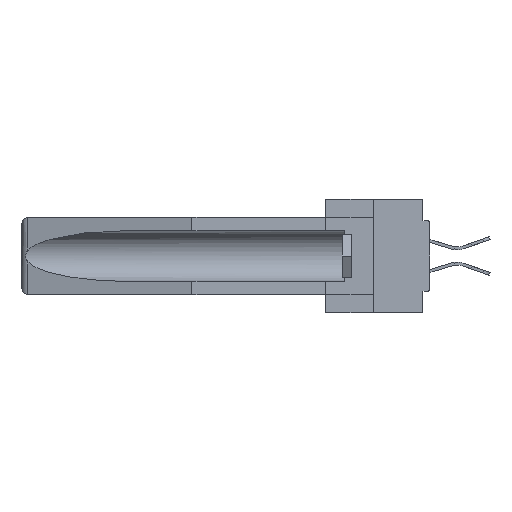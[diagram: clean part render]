
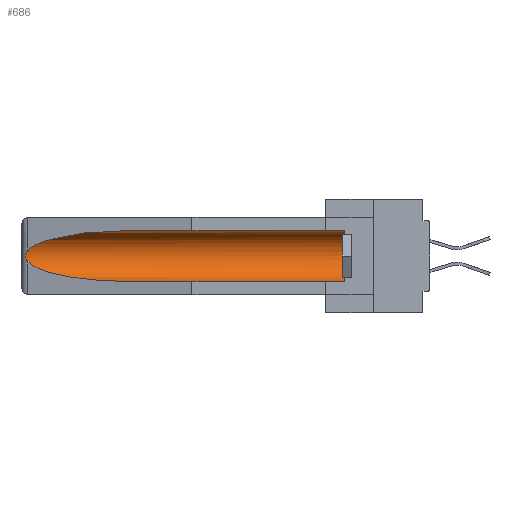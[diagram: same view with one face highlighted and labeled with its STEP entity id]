
A CAD part, left-side view. The second image highlights one B-rep face of the part: STEP entity #686.
In plain terms, the highlighted cylindrical face has radius 2.857 mm (diameter 5.715 mm), a partial arc.
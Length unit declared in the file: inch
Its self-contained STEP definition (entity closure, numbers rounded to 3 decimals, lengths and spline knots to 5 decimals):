
#209 = CARTESIAN_POINT ( 'NONE',  ( 0.21114, 1.30732, -0.059 ) ) ;
#418 = CARTESIAN_POINT ( 'NONE',  ( 0.155, 0.126, -0.059 ) ) ;
#686 = ADVANCED_FACE ( 'NONE', ( #12935 ), #26665, .F. ) ;
#3233 = VERTEX_POINT ( 'NONE', #4340 ) ;
#3239 = CARTESIAN_POINT ( 'NONE',  ( 0.26654, 1.53092, -0.15636 ) ) ;
#3310 = DIRECTION ( 'NONE',  ( 0., 0., 1. ) ) ;
#3386 = CARTESIAN_POINT ( 'NONE',  ( 0.26655, 1.53094, -0.18657 ) ) ;
#4313 = AXIS2_PLACEMENT_3D ( 'NONE', #39810, #33624, #14735 ) ;
#4340 = CARTESIAN_POINT ( 'NONE',  ( 0.26537, 1.52718, -0.14972 ) ) ;
#6380 = CARTESIAN_POINT ( 'NONE',  ( 0.155, 1.07973, -0.059 ) ) ;
#6397 = ORIENTED_EDGE ( 'NONE', *, *, #13262, .T. ) ;
#7364 = CIRCLE ( 'NONE', #10843, 0.1125 ) ;
#8047 = ORIENTED_EDGE ( 'NONE', *, *, #40123, .T. ) ;
#8463 = LINE ( 'NONE', #18401, #37579 ) ;
#8962 = EDGE_CURVE ( 'NONE', #23851, #27327, #7364, .T. ) ;
#9329 = CARTESIAN_POINT ( 'NONE',  ( 0.26537, 1.52718, -0.19328 ) ) ;
#10843 = AXIS2_PLACEMENT_3D ( 'NONE', #34357, #28221, #3310 ) ;
#12523 = LINE ( 'NONE', #21555, #29771 ) ;
#12935 = FACE_OUTER_BOUND ( 'NONE', #32820, .T. ) ;
#13262 = EDGE_CURVE ( 'NONE', #15906, #21639, #22846, .T. ) ;
#13336 = EDGE_CURVE ( 'NONE', #3233, #15906, #30739, .T. ) ;
#14735 = DIRECTION ( 'NONE',  ( 0., 0., 1. ) ) ;
#14847 =( BOUNDED_CURVE ( )  B_SPLINE_CURVE ( 3, ( #22648, #209, #16246, #29021 ),
 .UNSPECIFIED., .F., .F. ) 
 B_SPLINE_CURVE_WITH_KNOTS ( ( 4, 4 ),
 ( 4.71239, 6.08839 ),
 .UNSPECIFIED. ) 
 CURVE ( )  GEOMETRIC_REPRESENTATION_ITEM ( )  RATIONAL_B_SPLINE_CURVE ( ( 1., 0.848, 0.848, 1. ) ) 
 REPRESENTATION_ITEM ( '' )  );
#15262 = CARTESIAN_POINT ( 'NONE',  ( 0.26537, 1.52718, -0.14972 ) ) ;
#15906 = VERTEX_POINT ( 'NONE', #37518 ) ;
#16246 = CARTESIAN_POINT ( 'NONE',  ( 0.25451, 1.48313, -0.09465 ) ) ;
#18130 = CARTESIAN_POINT ( 'NONE',  ( 0.21114, 1.30732, -0.284 ) ) ;
#18401 = CARTESIAN_POINT ( 'NONE',  ( 0.155, -0.30754, -0.059 ) ) ;
#21134 = CARTESIAN_POINT ( 'NONE',  ( 0.26597, 1.52961, -0.15275 ) ) ;
#21330 = ORIENTED_EDGE ( 'NONE', *, *, #8962, .T. ) ;
#21555 = CARTESIAN_POINT ( 'NONE',  ( 0.155, -0.30754, -0.284 ) ) ;
#21639 = VERTEX_POINT ( 'NONE', #23959 ) ;
#22648 = CARTESIAN_POINT ( 'NONE',  ( 0.155, 1.07973, -0.059 ) ) ;
#22846 =( BOUNDED_CURVE ( )  B_SPLINE_CURVE ( 3, ( #34023, #34424, #18130, #28018 ),
 .UNSPECIFIED., .F., .F. ) 
 B_SPLINE_CURVE_WITH_KNOTS ( ( 4, 4 ),
 ( 0.1948, 1.5708 ),
 .UNSPECIFIED. ) 
 CURVE ( )  GEOMETRIC_REPRESENTATION_ITEM ( )  RATIONAL_B_SPLINE_CURVE ( ( 1., 0.848, 0.848, 1. ) ) 
 REPRESENTATION_ITEM ( '' )  );
#23152 = CARTESIAN_POINT ( 'NONE',  ( 0.155, 0.126, -0.284 ) ) ;
#23851 = VERTEX_POINT ( 'NONE', #23152 ) ;
#23959 = CARTESIAN_POINT ( 'NONE',  ( 0.155, 1.07973, -0.284 ) ) ;
#25394 = CARTESIAN_POINT ( 'NONE',  ( 0.2673, 1.5327, -0.16383 ) ) ;
#26462 = EDGE_CURVE ( 'NONE', #27104, #3233, #14847, .T. ) ;
#26665 = CYLINDRICAL_SURFACE ( 'NONE', #4313, 0.1125 ) ;
#27104 = VERTEX_POINT ( 'NONE', #6380 ) ;
#27327 = VERTEX_POINT ( 'NONE', #418 ) ;
#27500 = ORIENTED_EDGE ( 'NONE', *, *, #27562, .F. ) ;
#27562 = EDGE_CURVE ( 'NONE', #23851, #21639, #12523, .T. ) ;
#27646 = DIRECTION ( 'NONE',  ( 0., 1., 0. ) ) ;
#28018 = CARTESIAN_POINT ( 'NONE',  ( 0.155, 1.07973, -0.284 ) ) ;
#28221 = DIRECTION ( 'NONE',  ( 0., -1., 0. ) ) ;
#28718 = CARTESIAN_POINT ( 'NONE',  ( 0.26597, 1.5296, -0.19026 ) ) ;
#29020 = ORIENTED_EDGE ( 'NONE', *, *, #13336, .T. ) ;
#29021 = CARTESIAN_POINT ( 'NONE',  ( 0.26537, 1.52718, -0.14972 ) ) ;
#29771 = VECTOR ( 'NONE', #27646, 39.37008 ) ;
#30739 = B_SPLINE_CURVE_WITH_KNOTS ( 'NONE', 3,
 ( #15262, #21134, #3239, #25394, #31374, #35106, #37573, #3386, #28718, #9329 ),
 .UNSPECIFIED., .F., .F.,
 ( 4, 2, 2, 2, 4 ),
 ( 0., 0.00029, 0.00058, 0.00087, 0.00117 ),
 .UNSPECIFIED. ) ;
#31374 = CARTESIAN_POINT ( 'NONE',  ( 0.2675, 1.53308, -0.16763 ) ) ;
#32820 = EDGE_LOOP ( 'NONE', ( #34310, #29020, #6397, #27500, #21330, #8047 ) ) ;
#33624 = DIRECTION ( 'NONE',  ( 0., 1., 0. ) ) ;
#33894 = DIRECTION ( 'NONE',  ( 0., 1., 0. ) ) ;
#34023 = CARTESIAN_POINT ( 'NONE',  ( 0.26537, 1.52718, -0.19328 ) ) ;
#34310 = ORIENTED_EDGE ( 'NONE', *, *, #26462, .T. ) ;
#34357 = CARTESIAN_POINT ( 'NONE',  ( 0.155, 0.126, -0.1715 ) ) ;
#34424 = CARTESIAN_POINT ( 'NONE',  ( 0.25451, 1.48313, -0.24835 ) ) ;
#35106 = CARTESIAN_POINT ( 'NONE',  ( 0.2675, 1.53308, -0.17534 ) ) ;
#37518 = CARTESIAN_POINT ( 'NONE',  ( 0.26537, 1.52718, -0.19328 ) ) ;
#37573 = CARTESIAN_POINT ( 'NONE',  ( 0.2673, 1.53269, -0.17917 ) ) ;
#37579 = VECTOR ( 'NONE', #33894, 39.37008 ) ;
#39810 = CARTESIAN_POINT ( 'NONE',  ( 0.155, -0.30754, -0.1715 ) ) ;
#40123 = EDGE_CURVE ( 'NONE', #27327, #27104, #8463, .T. ) ;
